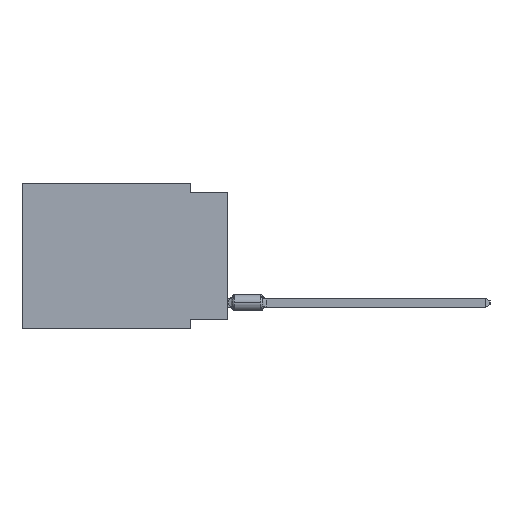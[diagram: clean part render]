
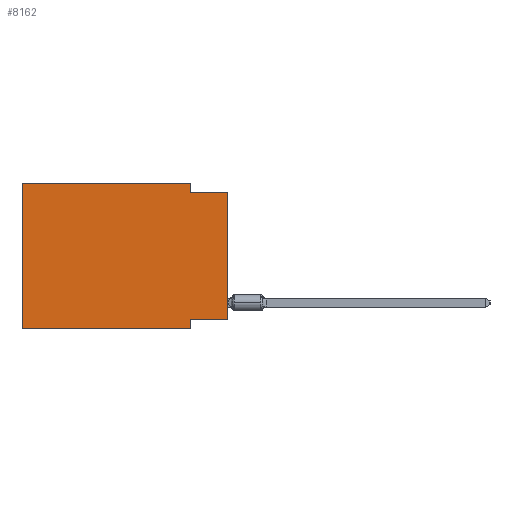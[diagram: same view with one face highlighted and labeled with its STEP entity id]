
A CAD part, left-side view. The second image highlights one B-rep face of the part: STEP entity #8162.
In plain terms, the highlighted planar face has unit normal (-1, 0, 0).
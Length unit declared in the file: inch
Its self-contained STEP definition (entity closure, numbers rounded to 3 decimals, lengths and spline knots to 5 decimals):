
#20 = CARTESIAN_POINT ( 'NONE',  ( 0., 0.1, -0.025 ) ) ;
#504 = LINE ( 'NONE', #9535, #3649 ) ;
#1704 = LINE ( 'NONE', #8422, #24332 ) ;
#2572 = CARTESIAN_POINT ( 'NONE',  ( 0., 0.1, -0.39 ) ) ;
#2794 = DIRECTION ( 'NONE',  ( 0., 0., -1. ) ) ;
#3649 = VECTOR ( 'NONE', #24252, 39.37008 ) ;
#3687 = ORIENTED_EDGE ( 'NONE', *, *, #7907, .F. ) ;
#3879 = VECTOR ( 'NONE', #10118, 39.37008 ) ;
#4511 = ORIENTED_EDGE ( 'NONE', *, *, #4817, .T. ) ;
#4817 = EDGE_CURVE ( 'NONE', #41609, #37279, #504, .T. ) ;
#5277 = CARTESIAN_POINT ( 'NONE',  ( 0., 0.55, -0.39 ) ) ;
#6810 = CARTESIAN_POINT ( 'NONE',  ( 0., 0.55, 0. ) ) ;
#6817 = CARTESIAN_POINT ( 'NONE',  ( 0., 0.55, 0. ) ) ;
#7907 = EDGE_CURVE ( 'NONE', #13335, #19448, #31942, .T. ) ;
#8162 = ADVANCED_FACE ( 'NONE', ( #44212 ), #37510, .F. ) ;
#8422 = CARTESIAN_POINT ( 'NONE',  ( 0., 0.55, -0.39 ) ) ;
#8622 = VECTOR ( 'NONE', #35306, 39.37008 ) ;
#9535 = CARTESIAN_POINT ( 'NONE',  ( 0., 0., 0. ) ) ;
#10118 = DIRECTION ( 'NONE',  ( 0., -1., 0. ) ) ;
#10502 = DIRECTION ( 'NONE',  ( 0., 1., 0. ) ) ;
#13266 = ORIENTED_EDGE ( 'NONE', *, *, #21367, .F. ) ;
#13335 = VERTEX_POINT ( 'NONE', #6810 ) ;
#14387 = EDGE_CURVE ( 'NONE', #42347, #28346, #33251, .T. ) ;
#16852 = DIRECTION ( 'NONE',  ( 0., 0., 1. ) ) ;
#17379 = VECTOR ( 'NONE', #10502, 39.37008 ) ;
#17650 = CARTESIAN_POINT ( 'NONE',  ( 0., 0., -0.365 ) ) ;
#19448 = VERTEX_POINT ( 'NONE', #21816 ) ;
#20371 = EDGE_LOOP ( 'NONE', ( #4511, #31648, #31653, #3687, #41182, #22823, #31293, #13266 ) ) ;
#21067 = LINE ( 'NONE', #34738, #3879 ) ;
#21367 = EDGE_CURVE ( 'NONE', #41609, #42347, #41202, .T. ) ;
#21636 = CARTESIAN_POINT ( 'NONE',  ( 0., 0.55, 0. ) ) ;
#21816 = CARTESIAN_POINT ( 'NONE',  ( 0., 0.1, 0. ) ) ;
#22823 = ORIENTED_EDGE ( 'NONE', *, *, #41823, .T. ) ;
#23351 = CARTESIAN_POINT ( 'NONE',  ( 0., 0.55, 0. ) ) ;
#23528 = VECTOR ( 'NONE', #42732, 39.37008 ) ;
#23596 = VECTOR ( 'NONE', #33239, 39.37008 ) ;
#23811 = LINE ( 'NONE', #23351, #25016 ) ;
#24252 = DIRECTION ( 'NONE',  ( 0., 0., 1. ) ) ;
#24332 = VECTOR ( 'NONE', #38899, 39.37008 ) ;
#25016 = VECTOR ( 'NONE', #16852, 39.37008 ) ;
#25513 = AXIS2_PLACEMENT_3D ( 'NONE', #6817, #33464, #2794 ) ;
#26341 = CARTESIAN_POINT ( 'NONE',  ( 0., 0., -0.365 ) ) ;
#28346 = VERTEX_POINT ( 'NONE', #33942 ) ;
#29843 = EDGE_CURVE ( 'NONE', #30764, #13335, #23811, .T. ) ;
#30306 = VERTEX_POINT ( 'NONE', #20 ) ;
#30764 = VERTEX_POINT ( 'NONE', #5277 ) ;
#30841 = EDGE_CURVE ( 'NONE', #19448, #30306, #43330, .T. ) ;
#31293 = ORIENTED_EDGE ( 'NONE', *, *, #14387, .F. ) ;
#31648 = ORIENTED_EDGE ( 'NONE', *, *, #36546, .F. ) ;
#31653 = ORIENTED_EDGE ( 'NONE', *, *, #30841, .F. ) ;
#31880 = CARTESIAN_POINT ( 'NONE',  ( 0., 0.1, -0.365 ) ) ;
#31942 = LINE ( 'NONE', #21636, #8622 ) ;
#33239 = DIRECTION ( 'NONE',  ( 0., 0., -1. ) ) ;
#33251 = LINE ( 'NONE', #2572, #23528 ) ;
#33464 = DIRECTION ( 'NONE',  ( 1., 0., 0. ) ) ;
#33942 = CARTESIAN_POINT ( 'NONE',  ( 0., 0.1, -0.39 ) ) ;
#34738 = CARTESIAN_POINT ( 'NONE',  ( 0., 0., -0.025 ) ) ;
#35306 = DIRECTION ( 'NONE',  ( 0., -1., 0. ) ) ;
#36546 = EDGE_CURVE ( 'NONE', #30306, #37279, #21067, .T. ) ;
#37279 = VERTEX_POINT ( 'NONE', #41303 ) ;
#37510 = PLANE ( 'NONE',  #25513 ) ;
#38899 = DIRECTION ( 'NONE',  ( 0., -1., 0. ) ) ;
#41182 = ORIENTED_EDGE ( 'NONE', *, *, #29843, .F. ) ;
#41202 = LINE ( 'NONE', #17650, #17379 ) ;
#41303 = CARTESIAN_POINT ( 'NONE',  ( 0., 0., -0.025 ) ) ;
#41609 = VERTEX_POINT ( 'NONE', #26341 ) ;
#41823 = EDGE_CURVE ( 'NONE', #30764, #28346, #1704, .T. ) ;
#42347 = VERTEX_POINT ( 'NONE', #31880 ) ;
#42732 = DIRECTION ( 'NONE',  ( 0., 0., -1. ) ) ;
#43111 = CARTESIAN_POINT ( 'NONE',  ( 0., 0.1, 0. ) ) ;
#43330 = LINE ( 'NONE', #43111, #23596 ) ;
#44212 = FACE_OUTER_BOUND ( 'NONE', #20371, .T. ) ;
